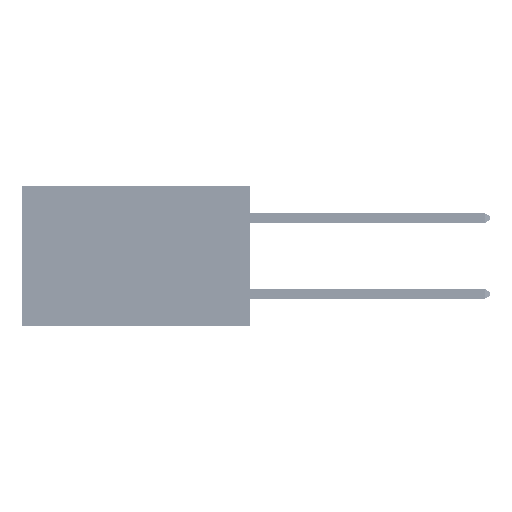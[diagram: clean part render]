
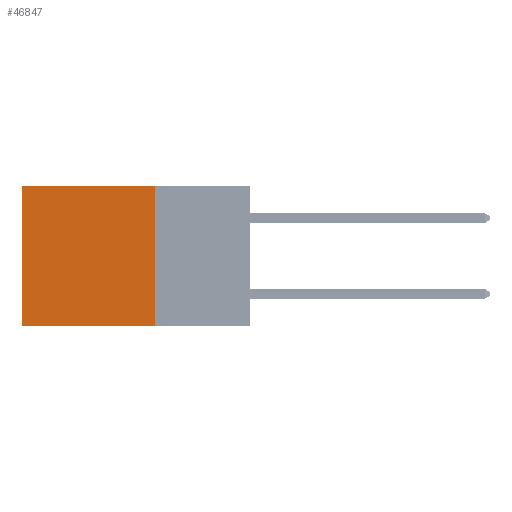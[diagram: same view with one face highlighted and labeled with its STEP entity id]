
A CAD part, left-side view. The second image highlights one B-rep face of the part: STEP entity #46847.
In plain terms, the highlighted planar face has unit normal (-1, 0, 0).
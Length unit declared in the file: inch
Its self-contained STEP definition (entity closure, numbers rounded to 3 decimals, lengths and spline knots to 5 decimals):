
#221 = ORIENTED_EDGE ( 'NONE', *, *, #41900, .T. ) ;
#1717 = CARTESIAN_POINT ( 'NONE',  ( 0.2875, 0.25, 0. ) ) ;
#6538 = CARTESIAN_POINT ( 'NONE',  ( 0.2875, 0.25, -0.37 ) ) ;
#7017 = EDGE_CURVE ( 'NONE', #44444, #26811, #18129, .T. ) ;
#7573 = VERTEX_POINT ( 'NONE', #26439 ) ;
#8272 = EDGE_CURVE ( 'NONE', #28835, #44444, #20328, .T. ) ;
#8555 = EDGE_CURVE ( 'NONE', #7573, #26811, #15681, .T. ) ;
#9556 = CARTESIAN_POINT ( 'NONE',  ( 0.2875, 0.25, 0. ) ) ;
#10491 = LINE ( 'NONE', #18207, #39376 ) ;
#12318 = CARTESIAN_POINT ( 'NONE',  ( 0.2875, 0.25, -0.37 ) ) ;
#13177 = FACE_OUTER_BOUND ( 'NONE', #13740, .T. ) ;
#13654 = CARTESIAN_POINT ( 'NONE',  ( 0.2875, 0.6, -0.37 ) ) ;
#13740 = EDGE_LOOP ( 'NONE', ( #39437, #42617, #39815, #221 ) ) ;
#15681 = LINE ( 'NONE', #37413, #27887 ) ;
#18129 = LINE ( 'NONE', #6538, #32401 ) ;
#18207 = CARTESIAN_POINT ( 'NONE',  ( 0.2875, 0.25, 0. ) ) ;
#19061 = DIRECTION ( 'NONE',  ( 0., 0., -1. ) ) ;
#20328 = LINE ( 'NONE', #1717, #21676 ) ;
#20643 = DIRECTION ( 'NONE',  ( 1., 0., 0. ) ) ;
#21676 = VECTOR ( 'NONE', #38915, 39.37008 ) ;
#24279 = DIRECTION ( 'NONE',  ( 0., 0., -1. ) ) ;
#26439 = CARTESIAN_POINT ( 'NONE',  ( 0.2875, 0.6, 0. ) ) ;
#26811 = VERTEX_POINT ( 'NONE', #13654 ) ;
#27887 = VECTOR ( 'NONE', #19061, 39.37008 ) ;
#27909 = PLANE ( 'NONE',  #30377 ) ;
#28835 = VERTEX_POINT ( 'NONE', #36742 ) ;
#30377 = AXIS2_PLACEMENT_3D ( 'NONE', #9556, #20643, #24279 ) ;
#32401 = VECTOR ( 'NONE', #39854, 39.37008 ) ;
#36742 = CARTESIAN_POINT ( 'NONE',  ( 0.2875, 0.25, 0. ) ) ;
#37413 = CARTESIAN_POINT ( 'NONE',  ( 0.2875, 0.6, 0. ) ) ;
#38915 = DIRECTION ( 'NONE',  ( 0., 0., -1. ) ) ;
#39376 = VECTOR ( 'NONE', #40631, 39.37008 ) ;
#39437 = ORIENTED_EDGE ( 'NONE', *, *, #8555, .T. ) ;
#39815 = ORIENTED_EDGE ( 'NONE', *, *, #8272, .F. ) ;
#39854 = DIRECTION ( 'NONE',  ( 0., 1., 0. ) ) ;
#40631 = DIRECTION ( 'NONE',  ( 0., 1., 0. ) ) ;
#41900 = EDGE_CURVE ( 'NONE', #28835, #7573, #10491, .T. ) ;
#42617 = ORIENTED_EDGE ( 'NONE', *, *, #7017, .F. ) ;
#44444 = VERTEX_POINT ( 'NONE', #12318 ) ;
#46847 = ADVANCED_FACE ( 'NONE', ( #13177 ), #27909, .F. ) ;
